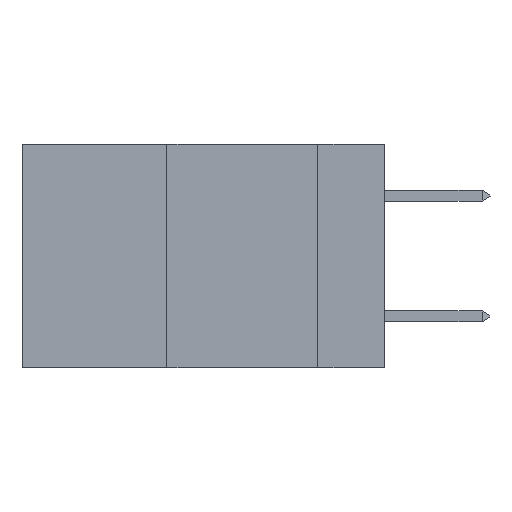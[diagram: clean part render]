
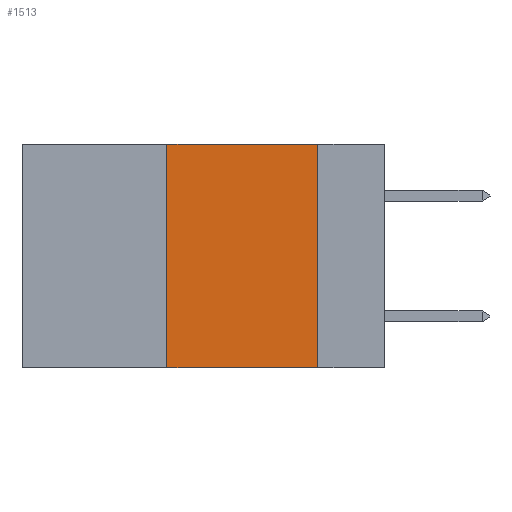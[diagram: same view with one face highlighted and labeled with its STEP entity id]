
A CAD part, left-side view. The second image highlights one B-rep face of the part: STEP entity #1513.
In plain terms, the highlighted planar face has unit normal (-1, 0, 0).
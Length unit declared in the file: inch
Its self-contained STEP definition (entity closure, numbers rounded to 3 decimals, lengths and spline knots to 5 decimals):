
#594 = CARTESIAN_POINT ( 'NONE',  ( 0., 0.11, 0. ) ) ;
#1513 = ADVANCED_FACE ( 'NONE', ( #20126 ), #9464, .F. ) ;
#2845 = CARTESIAN_POINT ( 'NONE',  ( 0., 0.6, -0.37 ) ) ;
#3805 = AXIS2_PLACEMENT_3D ( 'NONE', #18306, #9692, #11407 ) ;
#4385 = EDGE_CURVE ( 'NONE', #13225, #11428, #4948, .T. ) ;
#4948 = LINE ( 'NONE', #21294, #17715 ) ;
#5794 = VERTEX_POINT ( 'NONE', #9287 ) ;
#5934 = ORIENTED_EDGE ( 'NONE', *, *, #10306, .F. ) ;
#6091 = ORIENTED_EDGE ( 'NONE', *, *, #18460, .F. ) ;
#6127 = ORIENTED_EDGE ( 'NONE', *, *, #7754, .T. ) ;
#7051 = VECTOR ( 'NONE', #21606, 39.37008 ) ;
#7244 = VECTOR ( 'NONE', #22485, 39.37008 ) ;
#7544 = CARTESIAN_POINT ( 'NONE',  ( 0., 0.6, 0. ) ) ;
#7754 = EDGE_CURVE ( 'NONE', #5794, #11428, #11194, .T. ) ;
#8658 = LINE ( 'NONE', #10147, #7244 ) ;
#9287 = CARTESIAN_POINT ( 'NONE',  ( 0., 0.36, -0.37 ) ) ;
#9464 = PLANE ( 'NONE',  #3805 ) ;
#9692 = DIRECTION ( 'NONE',  ( 1., 0., 0. ) ) ;
#10147 = CARTESIAN_POINT ( 'NONE',  ( 0., 0.36, 0. ) ) ;
#10306 = EDGE_CURVE ( 'NONE', #5794, #10595, #8658, .T. ) ;
#10595 = VERTEX_POINT ( 'NONE', #17107 ) ;
#11194 = LINE ( 'NONE', #2845, #19283 ) ;
#11407 = DIRECTION ( 'NONE',  ( 0., 0., -1. ) ) ;
#11428 = VERTEX_POINT ( 'NONE', #21599 ) ;
#12570 = ORIENTED_EDGE ( 'NONE', *, *, #4385, .F. ) ;
#13225 = VERTEX_POINT ( 'NONE', #594 ) ;
#14637 = LINE ( 'NONE', #7544, #7051 ) ;
#16878 = EDGE_LOOP ( 'NONE', ( #12570, #6091, #5934, #6127 ) ) ;
#17107 = CARTESIAN_POINT ( 'NONE',  ( 0., 0.36, 0. ) ) ;
#17715 = VECTOR ( 'NONE', #18003, 39.37008 ) ;
#18003 = DIRECTION ( 'NONE',  ( 0., 0., -1. ) ) ;
#18306 = CARTESIAN_POINT ( 'NONE',  ( 0., 0.6, 0. ) ) ;
#18460 = EDGE_CURVE ( 'NONE', #10595, #13225, #14637, .T. ) ;
#19283 = VECTOR ( 'NONE', #21837, 39.37008 ) ;
#20126 = FACE_OUTER_BOUND ( 'NONE', #16878, .T. ) ;
#21294 = CARTESIAN_POINT ( 'NONE',  ( 0., 0.11, 0. ) ) ;
#21599 = CARTESIAN_POINT ( 'NONE',  ( 0., 0.11, -0.37 ) ) ;
#21606 = DIRECTION ( 'NONE',  ( 0., -1., 0. ) ) ;
#21837 = DIRECTION ( 'NONE',  ( 0., -1., 0. ) ) ;
#22485 = DIRECTION ( 'NONE',  ( 0., 0., 1. ) ) ;
